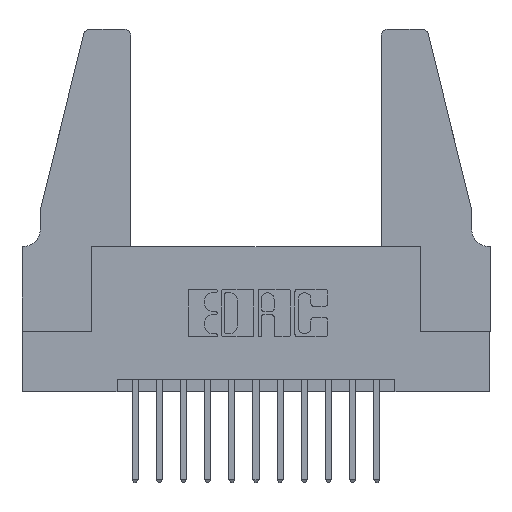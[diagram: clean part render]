
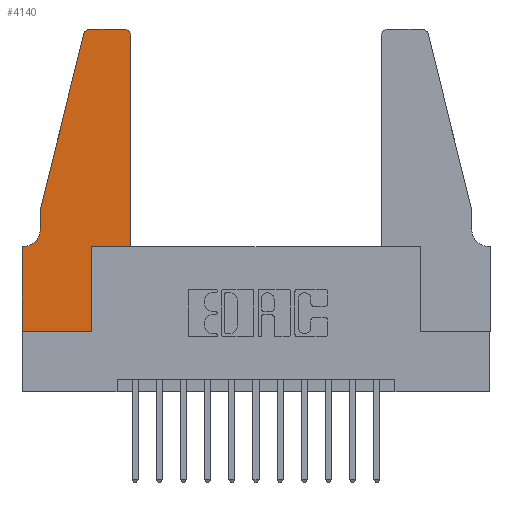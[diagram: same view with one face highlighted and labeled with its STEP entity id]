
A CAD part, top view. The second image highlights one B-rep face of the part: STEP entity #4140.
In plain terms, the highlighted planar face has unit normal (0, 0, 1).
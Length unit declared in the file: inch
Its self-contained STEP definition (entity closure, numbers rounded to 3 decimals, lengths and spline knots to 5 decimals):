
#1 = VECTOR ( 'NONE', #4155, 39.37008 ) ;
#55 = CARTESIAN_POINT ( 'NONE',  ( 0.0055, 0.42, 0.37 ) ) ;
#98 = VECTOR ( 'NONE', #6496, 39.37008 ) ;
#207 = ORIENTED_EDGE ( 'NONE', *, *, #12855, .T. ) ;
#533 = CARTESIAN_POINT ( 'NONE',  ( 0.2865, 0., 0.37 ) ) ;
#617 = EDGE_LOOP ( 'NONE', ( #10969, #6384, #13113, #207, #8479, #7199, #9033, #1295, #5594, #5962, #7955, #7710 ) ) ;
#1014 = VERTEX_POINT ( 'NONE', #8481 ) ;
#1056 = LINE ( 'NONE', #2822, #1 ) ;
#1100 = VERTEX_POINT ( 'NONE', #11346 ) ;
#1295 = ORIENTED_EDGE ( 'NONE', *, *, #14721, .T. ) ;
#1320 = CARTESIAN_POINT ( 'NONE',  ( 0., 0., 0.37 ) ) ;
#1332 = VECTOR ( 'NONE', #4064, 39.37008 ) ;
#1453 = VECTOR ( 'NONE', #11211, 39.37008 ) ;
#2525 = CARTESIAN_POINT ( 'NONE',  ( 0.0055, 0.35, 0.37 ) ) ;
#2669 = LINE ( 'NONE', #13270, #3235 ) ;
#2822 = CARTESIAN_POINT ( 'NONE',  ( 0., 0., 0.37 ) ) ;
#2829 = EDGE_CURVE ( 'NONE', #5597, #1100, #5284, .T. ) ;
#2985 = CIRCLE ( 'NONE', #8674, 0.03 ) ;
#3060 = CIRCLE ( 'NONE', #11705, 0.03 ) ;
#3127 = VERTEX_POINT ( 'NONE', #6080 ) ;
#3161 = CARTESIAN_POINT ( 'NONE',  ( 0.2865, 0.35, 0.37 ) ) ;
#3235 = VECTOR ( 'NONE', #6333, 39.37008 ) ;
#3477 = LINE ( 'NONE', #8912, #11839 ) ;
#4064 = DIRECTION ( 'NONE',  ( 0., -1., 0. ) ) ;
#4140 = ADVANCED_FACE ( 'NONE', ( #7041 ), #7274, .T. ) ;
#4155 = DIRECTION ( 'NONE',  ( 0., -1., 0. ) ) ;
#4168 = DIRECTION ( 'NONE',  ( 0., 1., 0. ) ) ;
#4203 = CARTESIAN_POINT ( 'NONE',  ( 0.4205, 1.25, 0.37 ) ) ;
#4457 = EDGE_CURVE ( 'NONE', #7606, #7547, #7982, .T. ) ;
#4535 = DIRECTION ( 'NONE',  ( 0., 0., 1. ) ) ;
#4559 = LINE ( 'NONE', #6459, #1453 ) ;
#4839 = VECTOR ( 'NONE', #13356, 39.37008 ) ;
#4879 = DIRECTION ( 'NONE',  ( 0., 1., 0. ) ) ;
#4947 = DIRECTION ( 'NONE',  ( 0., 0., 1. ) ) ;
#5110 = VERTEX_POINT ( 'NONE', #14393 ) ;
#5232 = VERTEX_POINT ( 'NONE', #4203 ) ;
#5284 = LINE ( 'NONE', #3161, #10374 ) ;
#5322 = EDGE_CURVE ( 'NONE', #1014, #7606, #6996, .T. ) ;
#5468 = EDGE_CURVE ( 'NONE', #3127, #6166, #2985, .T. ) ;
#5594 = ORIENTED_EDGE ( 'NONE', *, *, #2829, .T. ) ;
#5597 = VERTEX_POINT ( 'NONE', #533 ) ;
#5800 = EDGE_CURVE ( 'NONE', #6166, #7940, #7170, .T. ) ;
#5922 = CARTESIAN_POINT ( 'NONE',  ( 0., 0.35, 0.37 ) ) ;
#5962 = ORIENTED_EDGE ( 'NONE', *, *, #10685, .T. ) ;
#6080 = CARTESIAN_POINT ( 'NONE',  ( 0.284, 1.25, 0.37 ) ) ;
#6166 = VERTEX_POINT ( 'NONE', #10878 ) ;
#6333 = DIRECTION ( 'NONE',  ( -1., 0., 0. ) ) ;
#6343 = AXIS2_PLACEMENT_3D ( 'NONE', #55, #9334, #14795 ) ;
#6384 = ORIENTED_EDGE ( 'NONE', *, *, #5468, .T. ) ;
#6459 = CARTESIAN_POINT ( 'NONE',  ( 0., 0., 0.37 ) ) ;
#6496 = DIRECTION ( 'NONE',  ( -0.239, -0.971, 0. ) ) ;
#6996 = CIRCLE ( 'NONE', #6343, 0.07 ) ;
#7041 = FACE_OUTER_BOUND ( 'NONE', #617, .T. ) ;
#7103 = CARTESIAN_POINT ( 'NONE',  ( 0.284, 1.22, 0.37 ) ) ;
#7170 = LINE ( 'NONE', #14742, #98 ) ;
#7199 = ORIENTED_EDGE ( 'NONE', *, *, #4457, .T. ) ;
#7274 = PLANE ( 'NONE',  #11660 ) ;
#7319 = DIRECTION ( 'NONE',  ( 1., 0., 0. ) ) ;
#7547 = VERTEX_POINT ( 'NONE', #5922 ) ;
#7548 = CARTESIAN_POINT ( 'NONE',  ( 0.0755, 0.5, 0.37 ) ) ;
#7552 = CARTESIAN_POINT ( 'NONE',  ( 0.0755, 0.35, 0.37 ) ) ;
#7606 = VERTEX_POINT ( 'NONE', #2525 ) ;
#7710 = ORIENTED_EDGE ( 'NONE', *, *, #9325, .T. ) ;
#7940 = VERTEX_POINT ( 'NONE', #7548 ) ;
#7955 = ORIENTED_EDGE ( 'NONE', *, *, #13990, .T. ) ;
#7982 = LINE ( 'NONE', #7552, #4839 ) ;
#8288 = DIRECTION ( 'NONE',  ( 1., 0., 0. ) ) ;
#8479 = ORIENTED_EDGE ( 'NONE', *, *, #5322, .T. ) ;
#8481 = CARTESIAN_POINT ( 'NONE',  ( 0.0755, 0.42, 0.37 ) ) ;
#8674 = AXIS2_PLACEMENT_3D ( 'NONE', #7103, #4947, #8288 ) ;
#8912 = CARTESIAN_POINT ( 'NONE',  ( 0.4505, 0.35, 0.37 ) ) ;
#9017 = CARTESIAN_POINT ( 'NONE',  ( 0.4505, 0.35, 0.37 ) ) ;
#9033 = ORIENTED_EDGE ( 'NONE', *, *, #9729, .T. ) ;
#9073 = EDGE_CURVE ( 'NONE', #5232, #3127, #2669, .T. ) ;
#9124 = CARTESIAN_POINT ( 'NONE',  ( 0.4505, 0.35, 0.37 ) ) ;
#9325 = EDGE_CURVE ( 'NONE', #5110, #5232, #3060, .T. ) ;
#9334 = DIRECTION ( 'NONE',  ( 0., 0., -1. ) ) ;
#9596 = DIRECTION ( 'NONE',  ( 0., 0., 1. ) ) ;
#9729 = EDGE_CURVE ( 'NONE', #7547, #12672, #1056, .T. ) ;
#10374 = VECTOR ( 'NONE', #4879, 39.37008 ) ;
#10669 = DIRECTION ( 'NONE',  ( 1., 0., 0. ) ) ;
#10685 = EDGE_CURVE ( 'NONE', #1100, #13579, #14282, .T. ) ;
#10767 = CARTESIAN_POINT ( 'NONE',  ( 0., 0.35, 0.37 ) ) ;
#10846 = VECTOR ( 'NONE', #12622, 39.37008 ) ;
#10878 = CARTESIAN_POINT ( 'NONE',  ( 0.25487, 1.22718, 0.37 ) ) ;
#10969 = ORIENTED_EDGE ( 'NONE', *, *, #9073, .T. ) ;
#11211 = DIRECTION ( 'NONE',  ( 1., 0., 0. ) ) ;
#11346 = CARTESIAN_POINT ( 'NONE',  ( 0.2865, 0.35, 0.37 ) ) ;
#11487 = CARTESIAN_POINT ( 'NONE',  ( 0.4205, 1.22, 0.37 ) ) ;
#11660 = AXIS2_PLACEMENT_3D ( 'NONE', #10767, #9596, #7319 ) ;
#11705 = AXIS2_PLACEMENT_3D ( 'NONE', #11487, #4535, #10669 ) ;
#11839 = VECTOR ( 'NONE', #4168, 39.37008 ) ;
#12622 = DIRECTION ( 'NONE',  ( 1., 0., 0. ) ) ;
#12672 = VERTEX_POINT ( 'NONE', #1320 ) ;
#12855 = EDGE_CURVE ( 'NONE', #7940, #1014, #13165, .T. ) ;
#13113 = ORIENTED_EDGE ( 'NONE', *, *, #5800, .T. ) ;
#13165 = LINE ( 'NONE', #14523, #1332 ) ;
#13270 = CARTESIAN_POINT ( 'NONE',  ( 0.2605, 1.25, 0.37 ) ) ;
#13356 = DIRECTION ( 'NONE',  ( -1., 0., 0. ) ) ;
#13579 = VERTEX_POINT ( 'NONE', #9017 ) ;
#13990 = EDGE_CURVE ( 'NONE', #13579, #5110, #3477, .T. ) ;
#14282 = LINE ( 'NONE', #9124, #10846 ) ;
#14393 = CARTESIAN_POINT ( 'NONE',  ( 0.4505, 1.22, 0.37 ) ) ;
#14523 = CARTESIAN_POINT ( 'NONE',  ( 0.0755, 0.5, 0.37 ) ) ;
#14721 = EDGE_CURVE ( 'NONE', #12672, #5597, #4559, .T. ) ;
#14742 = CARTESIAN_POINT ( 'NONE',  ( 0.0755, 0.5, 0.37 ) ) ;
#14795 = DIRECTION ( 'NONE',  ( -1., 0., 0. ) ) ;
